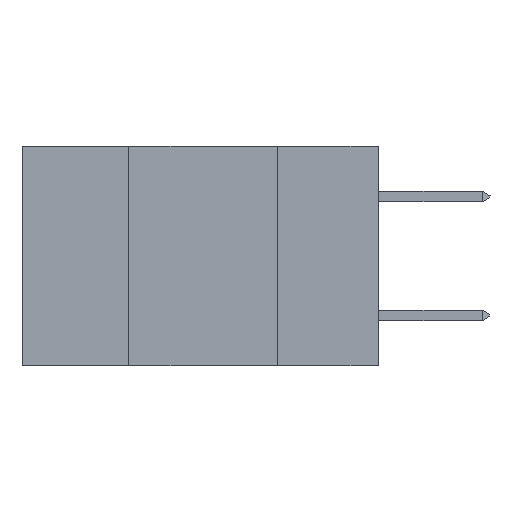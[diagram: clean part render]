
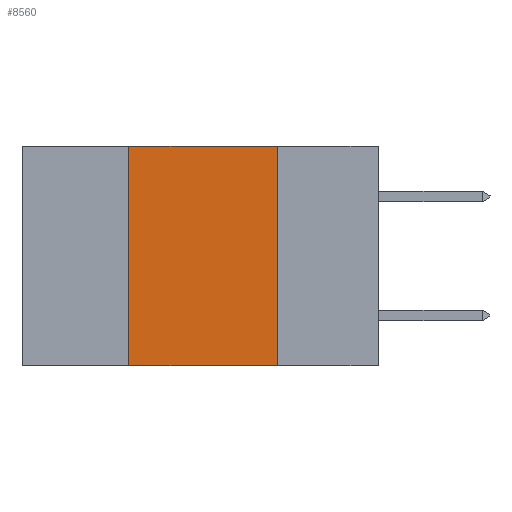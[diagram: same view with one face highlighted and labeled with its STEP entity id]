
A CAD part, left-side view. The second image highlights one B-rep face of the part: STEP entity #8560.
In plain terms, the highlighted planar face has unit normal (-1, 0, 0).
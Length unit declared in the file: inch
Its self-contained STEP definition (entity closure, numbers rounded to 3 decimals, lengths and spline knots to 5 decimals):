
#38 = EDGE_CURVE ( 'NONE', #2831, #18918, #9826, .T. ) ;
#888 = LINE ( 'NONE', #14655, #8105 ) ;
#1199 = ORIENTED_EDGE ( 'NONE', *, *, #2166, .F. ) ;
#2166 = EDGE_CURVE ( 'NONE', #18918, #19697, #12535, .T. ) ;
#2174 = AXIS2_PLACEMENT_3D ( 'NONE', #7688, #15067, #9390 ) ;
#2733 = CARTESIAN_POINT ( 'NONE',  ( 0., 0.6, 0. ) ) ;
#2831 = VERTEX_POINT ( 'NONE', #6064 ) ;
#2848 = DIRECTION ( 'NONE',  ( 0., -1., 0. ) ) ;
#4548 = LINE ( 'NONE', #11306, #13185 ) ;
#5279 = CARTESIAN_POINT ( 'NONE',  ( 0., 0.17, 0. ) ) ;
#6022 = CARTESIAN_POINT ( 'NONE',  ( 0., 0.42, -0.37 ) ) ;
#6064 = CARTESIAN_POINT ( 'NONE',  ( 0., 0.42, 0. ) ) ;
#6783 = ORIENTED_EDGE ( 'NONE', *, *, #16406, .T. ) ;
#7688 = CARTESIAN_POINT ( 'NONE',  ( 0., 0.6, 0. ) ) ;
#8014 = DIRECTION ( 'NONE',  ( 0., -1., 0. ) ) ;
#8105 = VECTOR ( 'NONE', #13064, 39.37008 ) ;
#8560 = ADVANCED_FACE ( 'NONE', ( #18212 ), #19715, .F. ) ;
#9170 = CARTESIAN_POINT ( 'NONE',  ( 0., 0.17, -0.37 ) ) ;
#9390 = DIRECTION ( 'NONE',  ( 0., 0., -1. ) ) ;
#9826 = LINE ( 'NONE', #2733, #15014 ) ;
#10950 = DIRECTION ( 'NONE',  ( 0., 0., -1. ) ) ;
#11306 = CARTESIAN_POINT ( 'NONE',  ( 0., 0.6, -0.37 ) ) ;
#12077 = EDGE_LOOP ( 'NONE', ( #1199, #20466, #13020, #6783 ) ) ;
#12324 = CARTESIAN_POINT ( 'NONE',  ( 0., 0.17, -0.37 ) ) ;
#12535 = LINE ( 'NONE', #12324, #18356 ) ;
#13020 = ORIENTED_EDGE ( 'NONE', *, *, #16047, .F. ) ;
#13064 = DIRECTION ( 'NONE',  ( 0., 0., 1. ) ) ;
#13185 = VECTOR ( 'NONE', #2848, 39.37008 ) ;
#14655 = CARTESIAN_POINT ( 'NONE',  ( 0., 0.42, -0.37 ) ) ;
#15014 = VECTOR ( 'NONE', #8014, 39.37008 ) ;
#15067 = DIRECTION ( 'NONE',  ( 1., 0., 0. ) ) ;
#16047 = EDGE_CURVE ( 'NONE', #19973, #2831, #888, .T. ) ;
#16406 = EDGE_CURVE ( 'NONE', #19973, #19697, #4548, .T. ) ;
#18212 = FACE_OUTER_BOUND ( 'NONE', #12077, .T. ) ;
#18356 = VECTOR ( 'NONE', #10950, 39.37008 ) ;
#18918 = VERTEX_POINT ( 'NONE', #5279 ) ;
#19697 = VERTEX_POINT ( 'NONE', #9170 ) ;
#19715 = PLANE ( 'NONE',  #2174 ) ;
#19973 = VERTEX_POINT ( 'NONE', #6022 ) ;
#20466 = ORIENTED_EDGE ( 'NONE', *, *, #38, .F. ) ;
